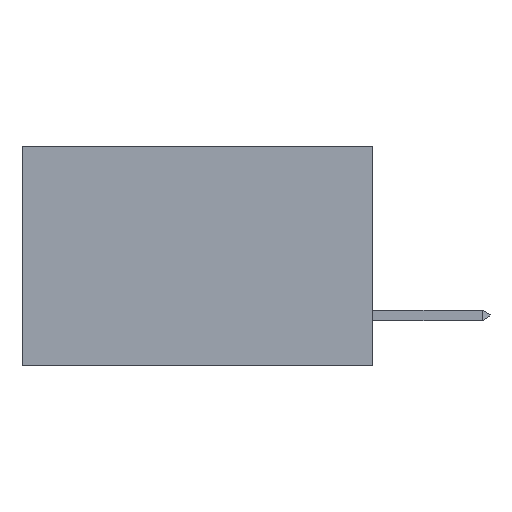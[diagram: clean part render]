
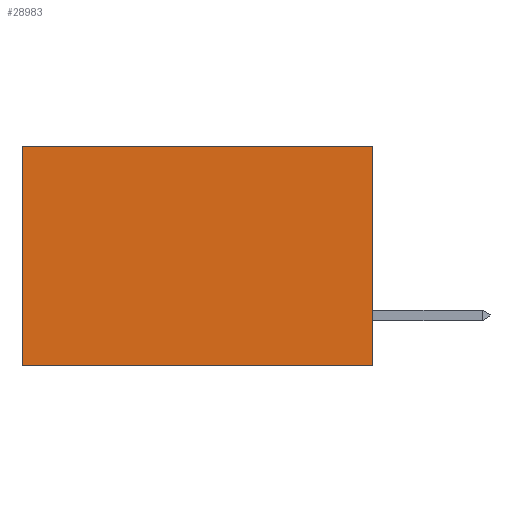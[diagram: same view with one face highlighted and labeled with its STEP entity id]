
A CAD part, left-side view. The second image highlights one B-rep face of the part: STEP entity #28983.
In plain terms, the highlighted planar face has unit normal (-1, 0, 0).
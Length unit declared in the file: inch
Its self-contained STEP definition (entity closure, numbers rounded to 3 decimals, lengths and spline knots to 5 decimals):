
#67 = LINE ( 'NONE', #6018, #10124 ) ;
#1151 = DIRECTION ( 'NONE',  ( 0., 0., -1. ) ) ;
#1357 = VERTEX_POINT ( 'NONE', #25274 ) ;
#3049 = ORIENTED_EDGE ( 'NONE', *, *, #6582, .T. ) ;
#4431 = LINE ( 'NONE', #25776, #15747 ) ;
#4445 = EDGE_CURVE ( 'NONE', #11029, #5040, #67, .T. ) ;
#5040 = VERTEX_POINT ( 'NONE', #12636 ) ;
#5346 = VECTOR ( 'NONE', #24534, 39.37008 ) ;
#5596 = CARTESIAN_POINT ( 'NONE',  ( 0.277, 0., 0. ) ) ;
#5984 = DIRECTION ( 'NONE',  ( 0., 1., 0. ) ) ;
#6018 = CARTESIAN_POINT ( 'NONE',  ( 0.277, 0., -0.37 ) ) ;
#6582 = EDGE_CURVE ( 'NONE', #1357, #5040, #23282, .T. ) ;
#6644 = EDGE_LOOP ( 'NONE', ( #3049, #6941, #9070, #23269 ) ) ;
#6941 = ORIENTED_EDGE ( 'NONE', *, *, #4445, .F. ) ;
#9070 = ORIENTED_EDGE ( 'NONE', *, *, #26944, .F. ) ;
#9181 = CARTESIAN_POINT ( 'NONE',  ( 0.277, 0., -0.37 ) ) ;
#10124 = VECTOR ( 'NONE', #5984, 39.37008 ) ;
#10272 = PLANE ( 'NONE',  #24672 ) ;
#10765 = VERTEX_POINT ( 'NONE', #5596 ) ;
#11029 = VERTEX_POINT ( 'NONE', #9181 ) ;
#12552 = VECTOR ( 'NONE', #18723, 39.37008 ) ;
#12636 = CARTESIAN_POINT ( 'NONE',  ( 0.277, 0.59, -0.37 ) ) ;
#14202 = FACE_OUTER_BOUND ( 'NONE', #6644, .T. ) ;
#14589 = DIRECTION ( 'NONE',  ( 0., 1., 0. ) ) ;
#14763 = DIRECTION ( 'NONE',  ( 1., 0., 0. ) ) ;
#15747 = VECTOR ( 'NONE', #14589, 39.37008 ) ;
#16513 = CARTESIAN_POINT ( 'NONE',  ( 0.277, 0., -0.37 ) ) ;
#18723 = DIRECTION ( 'NONE',  ( 0., 0., -1. ) ) ;
#19748 = EDGE_CURVE ( 'NONE', #10765, #1357, #4431, .T. ) ;
#23269 = ORIENTED_EDGE ( 'NONE', *, *, #19748, .T. ) ;
#23282 = LINE ( 'NONE', #24162, #5346 ) ;
#24162 = CARTESIAN_POINT ( 'NONE',  ( 0.277, 0.59, -0.37 ) ) ;
#24473 = LINE ( 'NONE', #16513, #12552 ) ;
#24534 = DIRECTION ( 'NONE',  ( 0., 0., -1. ) ) ;
#24672 = AXIS2_PLACEMENT_3D ( 'NONE', #28195, #14763, #1151 ) ;
#25274 = CARTESIAN_POINT ( 'NONE',  ( 0.277, 0.59, 0. ) ) ;
#25776 = CARTESIAN_POINT ( 'NONE',  ( 0.277, 0., 0. ) ) ;
#26944 = EDGE_CURVE ( 'NONE', #10765, #11029, #24473, .T. ) ;
#28195 = CARTESIAN_POINT ( 'NONE',  ( 0.277, 0., -0.37 ) ) ;
#28983 = ADVANCED_FACE ( 'NONE', ( #14202 ), #10272, .F. ) ;
